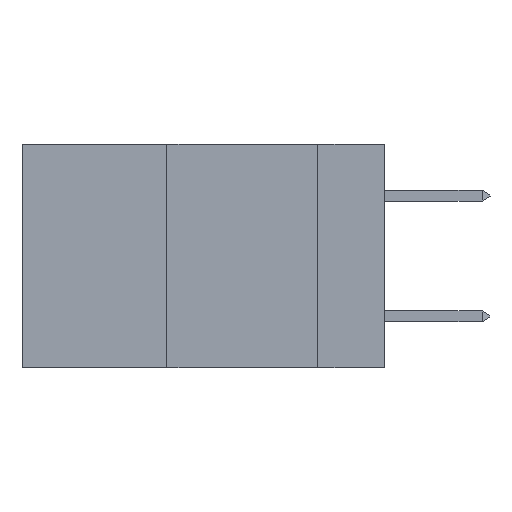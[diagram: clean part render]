
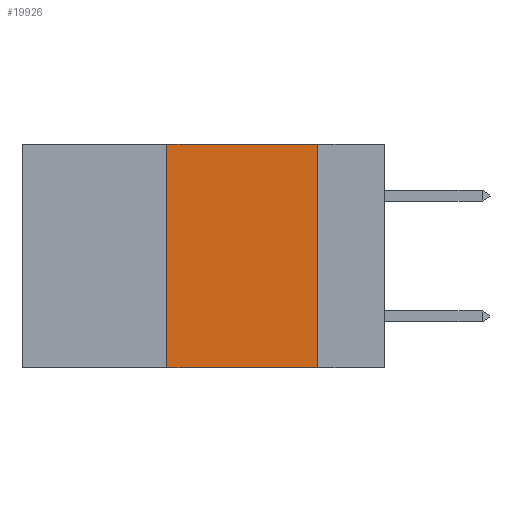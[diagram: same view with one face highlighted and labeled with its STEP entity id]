
A CAD part, left-side view. The second image highlights one B-rep face of the part: STEP entity #19926.
In plain terms, the highlighted planar face has unit normal (-1, 0, 0).
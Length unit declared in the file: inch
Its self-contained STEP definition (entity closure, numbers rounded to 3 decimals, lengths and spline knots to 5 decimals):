
#112 = FACE_OUTER_BOUND ( 'NONE', #22460, .T. ) ;
#1960 = DIRECTION ( 'NONE',  ( 0., 0., -1. ) ) ;
#2023 = AXIS2_PLACEMENT_3D ( 'NONE', #14627, #11229, #20302 ) ;
#2203 = ORIENTED_EDGE ( 'NONE', *, *, #7896, .T. ) ;
#2345 = LINE ( 'NONE', #20619, #21138 ) ;
#2915 = LINE ( 'NONE', #11981, #20196 ) ;
#4058 = EDGE_CURVE ( 'NONE', #7949, #14717, #11060, .T. ) ;
#4467 = ORIENTED_EDGE ( 'NONE', *, *, #13557, .F. ) ;
#4724 = DIRECTION ( 'NONE',  ( 0., -1., 0. ) ) ;
#6498 = CARTESIAN_POINT ( 'NONE',  ( 0., 0.11, -0.37 ) ) ;
#7896 = EDGE_CURVE ( 'NONE', #7949, #8286, #2915, .T. ) ;
#7949 = VERTEX_POINT ( 'NONE', #14042 ) ;
#8286 = VERTEX_POINT ( 'NONE', #6498 ) ;
#11060 = LINE ( 'NONE', #18414, #21652 ) ;
#11229 = DIRECTION ( 'NONE',  ( 1., 0., 0. ) ) ;
#11519 = VERTEX_POINT ( 'NONE', #22025 ) ;
#11552 = VECTOR ( 'NONE', #1960, 39.37008 ) ;
#11981 = CARTESIAN_POINT ( 'NONE',  ( 0., 0.6, -0.37 ) ) ;
#13049 = PLANE ( 'NONE',  #2023 ) ;
#13442 = CARTESIAN_POINT ( 'NONE',  ( 0., 0.11, 0. ) ) ;
#13557 = EDGE_CURVE ( 'NONE', #14717, #11519, #2345, .T. ) ;
#14042 = CARTESIAN_POINT ( 'NONE',  ( 0., 0.36, -0.37 ) ) ;
#14627 = CARTESIAN_POINT ( 'NONE',  ( 0., 0.6, 0. ) ) ;
#14717 = VERTEX_POINT ( 'NONE', #20132 ) ;
#15131 = LINE ( 'NONE', #13442, #11552 ) ;
#15287 = DIRECTION ( 'NONE',  ( 0., -1., 0. ) ) ;
#16651 = EDGE_CURVE ( 'NONE', #11519, #8286, #15131, .T. ) ;
#18414 = CARTESIAN_POINT ( 'NONE',  ( 0., 0.36, 0. ) ) ;
#19926 = ADVANCED_FACE ( 'NONE', ( #112 ), #13049, .F. ) ;
#20132 = CARTESIAN_POINT ( 'NONE',  ( 0., 0.36, 0. ) ) ;
#20196 = VECTOR ( 'NONE', #4724, 39.37008 ) ;
#20302 = DIRECTION ( 'NONE',  ( 0., 0., -1. ) ) ;
#20619 = CARTESIAN_POINT ( 'NONE',  ( 0., 0.6, 0. ) ) ;
#21000 = ORIENTED_EDGE ( 'NONE', *, *, #16651, .F. ) ;
#21138 = VECTOR ( 'NONE', #15287, 39.37008 ) ;
#21652 = VECTOR ( 'NONE', #22892, 39.37008 ) ;
#22025 = CARTESIAN_POINT ( 'NONE',  ( 0., 0.11, 0. ) ) ;
#22460 = EDGE_LOOP ( 'NONE', ( #21000, #4467, #23463, #2203 ) ) ;
#22892 = DIRECTION ( 'NONE',  ( 0., 0., 1. ) ) ;
#23463 = ORIENTED_EDGE ( 'NONE', *, *, #4058, .F. ) ;
